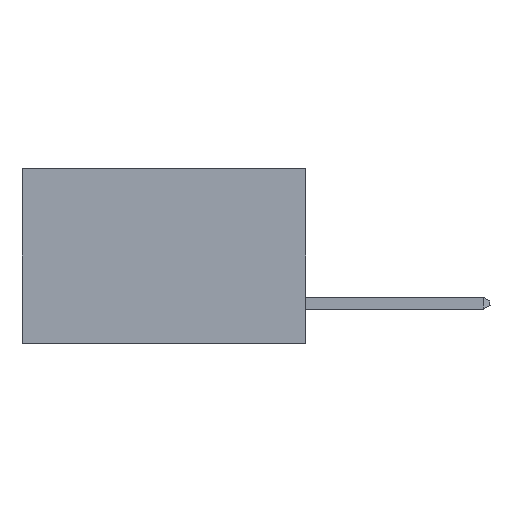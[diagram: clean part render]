
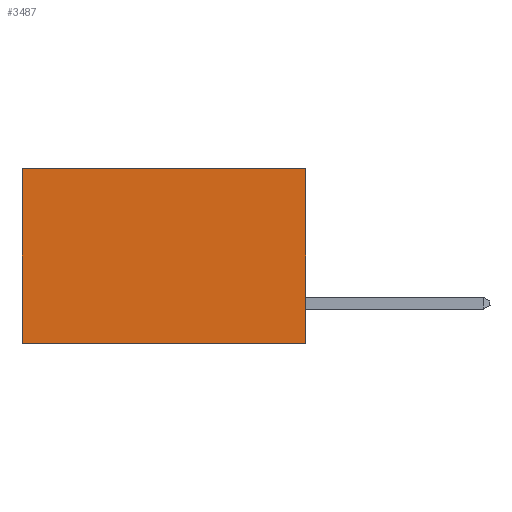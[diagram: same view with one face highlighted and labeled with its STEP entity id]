
A CAD part, left-side view. The second image highlights one B-rep face of the part: STEP entity #3487.
In plain terms, the highlighted planar face has unit normal (-1, 0, 0).
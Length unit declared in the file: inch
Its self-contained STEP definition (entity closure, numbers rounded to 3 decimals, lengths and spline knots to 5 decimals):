
#721 = DIRECTION ( 'NONE',  ( 0., 0., -1. ) ) ;
#866 = DIRECTION ( 'NONE',  ( 1., 0., 0. ) ) ;
#2538 = CARTESIAN_POINT ( 'NONE',  ( 0.298, 0.6, 0. ) ) ;
#3034 = CARTESIAN_POINT ( 'NONE',  ( 0.298, 0.6, -0.37 ) ) ;
#3197 = DIRECTION ( 'NONE',  ( 0., 1., 0. ) ) ;
#3487 = ADVANCED_FACE ( 'NONE', ( #11601 ), #16737, .F. ) ;
#5033 = ORIENTED_EDGE ( 'NONE', *, *, #13986, .T. ) ;
#6546 = VERTEX_POINT ( 'NONE', #10244 ) ;
#6842 = LINE ( 'NONE', #12996, #10563 ) ;
#7496 = ORIENTED_EDGE ( 'NONE', *, *, #8381, .F. ) ;
#7589 = LINE ( 'NONE', #15248, #11576 ) ;
#7607 = EDGE_CURVE ( 'NONE', #10514, #8494, #7589, .T. ) ;
#7887 = EDGE_CURVE ( 'NONE', #6546, #19777, #6842, .T. ) ;
#8241 = EDGE_LOOP ( 'NONE', ( #5033, #19071, #7496, #14958 ) ) ;
#8381 = EDGE_CURVE ( 'NONE', #6546, #10514, #17015, .T. ) ;
#8494 = VERTEX_POINT ( 'NONE', #3034 ) ;
#10244 = CARTESIAN_POINT ( 'NONE',  ( 0.298, 0., 0. ) ) ;
#10514 = VERTEX_POINT ( 'NONE', #13493 ) ;
#10563 = VECTOR ( 'NONE', #3197, 39.37008 ) ;
#11576 = VECTOR ( 'NONE', #13666, 39.37008 ) ;
#11601 = FACE_OUTER_BOUND ( 'NONE', #8241, .T. ) ;
#12996 = CARTESIAN_POINT ( 'NONE',  ( 0.298, 0., 0. ) ) ;
#13313 = VECTOR ( 'NONE', #17287, 39.37008 ) ;
#13493 = CARTESIAN_POINT ( 'NONE',  ( 0.298, 0., -0.37 ) ) ;
#13666 = DIRECTION ( 'NONE',  ( 0., 1., 0. ) ) ;
#13986 = EDGE_CURVE ( 'NONE', #19777, #8494, #14701, .T. ) ;
#14176 = CARTESIAN_POINT ( 'NONE',  ( 0.298, 0.6, 0. ) ) ;
#14378 = DIRECTION ( 'NONE',  ( 0., 0., -1. ) ) ;
#14701 = LINE ( 'NONE', #14176, #20115 ) ;
#14958 = ORIENTED_EDGE ( 'NONE', *, *, #7887, .T. ) ;
#15248 = CARTESIAN_POINT ( 'NONE',  ( 0.298, 0., -0.37 ) ) ;
#16737 = PLANE ( 'NONE',  #19849 ) ;
#17015 = LINE ( 'NONE', #17489, #13313 ) ;
#17287 = DIRECTION ( 'NONE',  ( 0., 0., -1. ) ) ;
#17489 = CARTESIAN_POINT ( 'NONE',  ( 0.298, 0., 0. ) ) ;
#18128 = CARTESIAN_POINT ( 'NONE',  ( 0.298, 0., 0. ) ) ;
#19071 = ORIENTED_EDGE ( 'NONE', *, *, #7607, .F. ) ;
#19777 = VERTEX_POINT ( 'NONE', #2538 ) ;
#19849 = AXIS2_PLACEMENT_3D ( 'NONE', #18128, #866, #721 ) ;
#20115 = VECTOR ( 'NONE', #14378, 39.37008 ) ;
